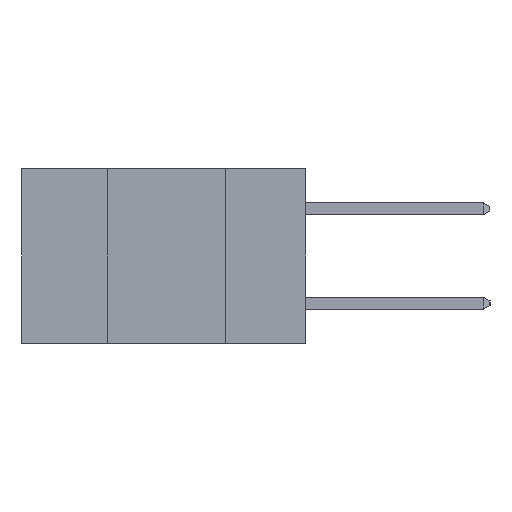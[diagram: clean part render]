
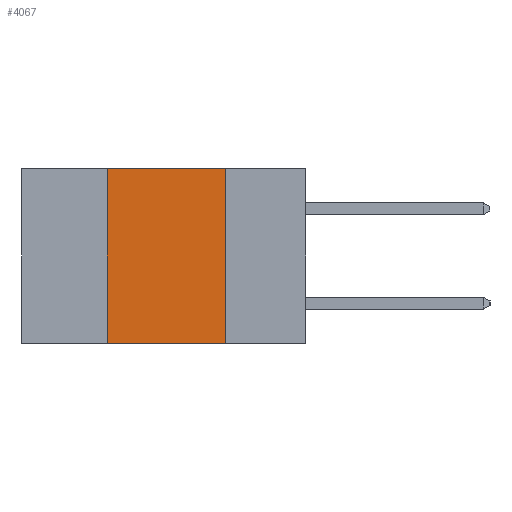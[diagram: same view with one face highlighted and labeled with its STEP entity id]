
A CAD part, left-side view. The second image highlights one B-rep face of the part: STEP entity #4067.
In plain terms, the highlighted planar face has unit normal (-1, 0, 0).
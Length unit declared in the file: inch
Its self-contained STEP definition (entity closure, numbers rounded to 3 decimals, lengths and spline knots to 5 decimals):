
#324 = EDGE_CURVE ( 'NONE', #6273, #6326, #10170, .T. ) ;
#650 = CARTESIAN_POINT ( 'NONE',  ( 0., 0.6, -0.37 ) ) ;
#670 = VERTEX_POINT ( 'NONE', #4540 ) ;
#1042 = ORIENTED_EDGE ( 'NONE', *, *, #11740, .F. ) ;
#1191 = CARTESIAN_POINT ( 'NONE',  ( 0., 0.42, -0.37 ) ) ;
#1685 = FACE_OUTER_BOUND ( 'NONE', #6404, .T. ) ;
#1737 = VECTOR ( 'NONE', #6496, 39.37008 ) ;
#2779 = DIRECTION ( 'NONE',  ( 0., -1., 0. ) ) ;
#3108 = CARTESIAN_POINT ( 'NONE',  ( 0., 0.17, -0.37 ) ) ;
#3695 = CARTESIAN_POINT ( 'NONE',  ( 0., 0.42, -0.37 ) ) ;
#4067 = ADVANCED_FACE ( 'NONE', ( #1685 ), #12670, .F. ) ;
#4281 = VECTOR ( 'NONE', #6381, 39.37008 ) ;
#4540 = CARTESIAN_POINT ( 'NONE',  ( 0., 0.42, 0. ) ) ;
#4823 = VECTOR ( 'NONE', #2779, 39.37008 ) ;
#4981 = LINE ( 'NONE', #7372, #4281 ) ;
#5750 = ORIENTED_EDGE ( 'NONE', *, *, #324, .T. ) ;
#6273 = VERTEX_POINT ( 'NONE', #3695 ) ;
#6326 = VERTEX_POINT ( 'NONE', #3108 ) ;
#6381 = DIRECTION ( 'NONE',  ( 0., 0., -1. ) ) ;
#6404 = EDGE_LOOP ( 'NONE', ( #1042, #11054, #7291, #5750 ) ) ;
#6496 = DIRECTION ( 'NONE',  ( 0., 0., 1. ) ) ;
#7291 = ORIENTED_EDGE ( 'NONE', *, *, #12986, .F. ) ;
#7355 = CARTESIAN_POINT ( 'NONE',  ( 0., 0.6, 0. ) ) ;
#7372 = CARTESIAN_POINT ( 'NONE',  ( 0., 0.17, -0.37 ) ) ;
#7491 = VECTOR ( 'NONE', #8387, 39.37008 ) ;
#8369 = CARTESIAN_POINT ( 'NONE',  ( 0., 0.17, 0. ) ) ;
#8387 = DIRECTION ( 'NONE',  ( 0., -1., 0. ) ) ;
#9595 = VERTEX_POINT ( 'NONE', #8369 ) ;
#9971 = LINE ( 'NONE', #1191, #1737 ) ;
#10170 = LINE ( 'NONE', #650, #4823 ) ;
#11054 = ORIENTED_EDGE ( 'NONE', *, *, #12371, .F. ) ;
#11380 = AXIS2_PLACEMENT_3D ( 'NONE', #12561, #12527, #12524 ) ;
#11740 = EDGE_CURVE ( 'NONE', #9595, #6326, #4981, .T. ) ;
#12371 = EDGE_CURVE ( 'NONE', #670, #9595, #12792, .T. ) ;
#12524 = DIRECTION ( 'NONE',  ( 0., 0., -1. ) ) ;
#12527 = DIRECTION ( 'NONE',  ( 1., 0., 0. ) ) ;
#12561 = CARTESIAN_POINT ( 'NONE',  ( 0., 0.6, 0. ) ) ;
#12670 = PLANE ( 'NONE',  #11380 ) ;
#12792 = LINE ( 'NONE', #7355, #7491 ) ;
#12986 = EDGE_CURVE ( 'NONE', #6273, #670, #9971, .T. ) ;
